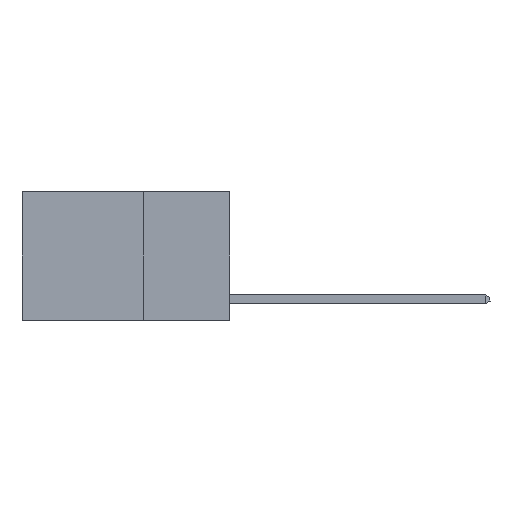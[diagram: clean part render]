
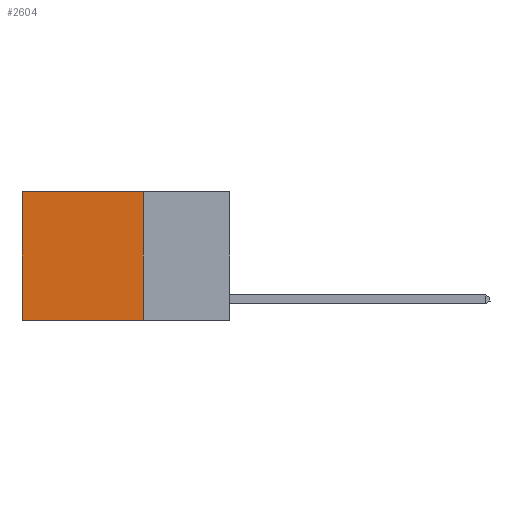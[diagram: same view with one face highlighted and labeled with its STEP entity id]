
A CAD part, left-side view. The second image highlights one B-rep face of the part: STEP entity #2604.
In plain terms, the highlighted planar face has unit normal (-1, 0, 0).
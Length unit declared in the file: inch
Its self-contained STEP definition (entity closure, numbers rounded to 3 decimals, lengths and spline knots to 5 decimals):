
#940 = VERTEX_POINT ( 'NONE', #7139 ) ;
#1284 = VECTOR ( 'NONE', #2515, 39.37008 ) ;
#1476 = VECTOR ( 'NONE', #10791, 39.37008 ) ;
#1487 = CARTESIAN_POINT ( 'NONE',  ( 0.2625, 0.25, 0. ) ) ;
#1712 = FACE_OUTER_BOUND ( 'NONE', #4565, .T. ) ;
#1984 = LINE ( 'NONE', #5092, #11178 ) ;
#2370 = CARTESIAN_POINT ( 'NONE',  ( 0.2625, 0.25, 0. ) ) ;
#2515 = DIRECTION ( 'NONE',  ( 0., 1., 0. ) ) ;
#2591 = VERTEX_POINT ( 'NONE', #2977 ) ;
#2604 = ADVANCED_FACE ( 'NONE', ( #1712 ), #9349, .F. ) ;
#2638 = DIRECTION ( 'NONE',  ( 0., 1., 0. ) ) ;
#2710 = VERTEX_POINT ( 'NONE', #2370 ) ;
#2745 = EDGE_CURVE ( 'NONE', #2710, #2591, #7917, .T. ) ;
#2977 = CARTESIAN_POINT ( 'NONE',  ( 0.2625, 0.6, 0. ) ) ;
#3003 = ORIENTED_EDGE ( 'NONE', *, *, #7714, .T. ) ;
#3555 = VERTEX_POINT ( 'NONE', #8570 ) ;
#4045 = DIRECTION ( 'NONE',  ( 1., 0., 0. ) ) ;
#4231 = EDGE_CURVE ( 'NONE', #2710, #940, #1984, .T. ) ;
#4565 = EDGE_LOOP ( 'NONE', ( #3003, #5544, #8157, #10513 ) ) ;
#5092 = CARTESIAN_POINT ( 'NONE',  ( 0.2625, 0.25, 0. ) ) ;
#5509 = CARTESIAN_POINT ( 'NONE',  ( 0.2625, 0.6, 0. ) ) ;
#5544 = ORIENTED_EDGE ( 'NONE', *, *, #7734, .F. ) ;
#6830 = DIRECTION ( 'NONE',  ( 0., 0., -1. ) ) ;
#7139 = CARTESIAN_POINT ( 'NONE',  ( 0.2625, 0.25, -0.37 ) ) ;
#7245 = CARTESIAN_POINT ( 'NONE',  ( 0.2625, 0.25, -0.37 ) ) ;
#7600 = CARTESIAN_POINT ( 'NONE',  ( 0.2625, 0.25, 0. ) ) ;
#7714 = EDGE_CURVE ( 'NONE', #2591, #3555, #8906, .T. ) ;
#7734 = EDGE_CURVE ( 'NONE', #940, #3555, #11267, .T. ) ;
#7917 = LINE ( 'NONE', #1487, #1284 ) ;
#8157 = ORIENTED_EDGE ( 'NONE', *, *, #4231, .F. ) ;
#8570 = CARTESIAN_POINT ( 'NONE',  ( 0.2625, 0.6, -0.37 ) ) ;
#8906 = LINE ( 'NONE', #5509, #1476 ) ;
#9349 = PLANE ( 'NONE',  #10426 ) ;
#10265 = DIRECTION ( 'NONE',  ( 0., 0., -1. ) ) ;
#10426 = AXIS2_PLACEMENT_3D ( 'NONE', #7600, #4045, #10265 ) ;
#10513 = ORIENTED_EDGE ( 'NONE', *, *, #2745, .T. ) ;
#10791 = DIRECTION ( 'NONE',  ( 0., 0., -1. ) ) ;
#10993 = VECTOR ( 'NONE', #2638, 39.37008 ) ;
#11178 = VECTOR ( 'NONE', #6830, 39.37008 ) ;
#11267 = LINE ( 'NONE', #7245, #10993 ) ;
